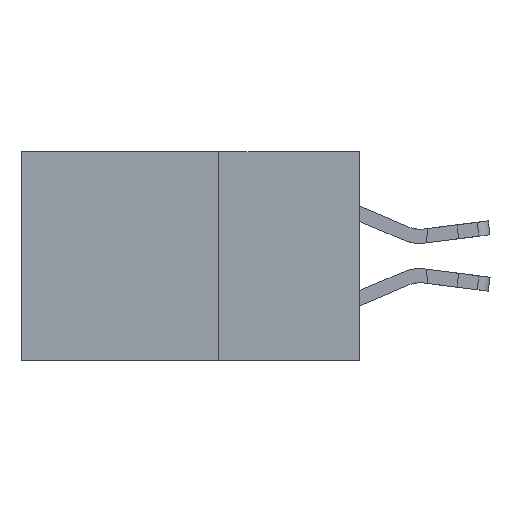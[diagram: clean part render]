
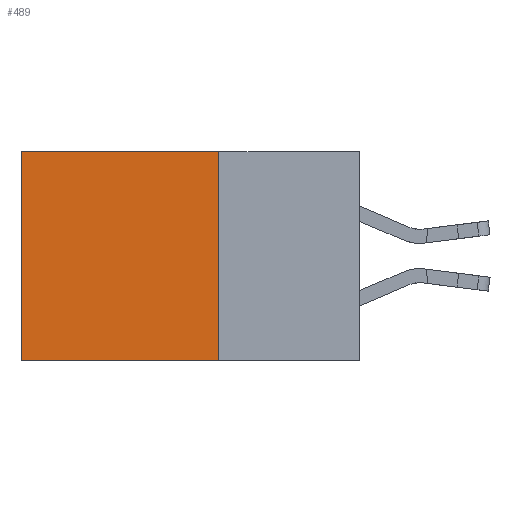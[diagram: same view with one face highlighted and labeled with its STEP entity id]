
A CAD part, left-side view. The second image highlights one B-rep face of the part: STEP entity #489.
In plain terms, the highlighted planar face has unit normal (-1, 0, 0).
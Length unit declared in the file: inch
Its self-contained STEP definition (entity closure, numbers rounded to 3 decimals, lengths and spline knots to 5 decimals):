
#489 = ADVANCED_FACE ( 'NONE', ( #14061 ), #24746, .F. ) ;
#1127 = VERTEX_POINT ( 'NONE', #13816 ) ;
#1723 = CARTESIAN_POINT ( 'NONE',  ( 0.2875, 0.6, -0.37 ) ) ;
#1935 = EDGE_CURVE ( 'NONE', #1127, #5653, #5697, .T. ) ;
#2310 = VERTEX_POINT ( 'NONE', #27118 ) ;
#2506 = CARTESIAN_POINT ( 'NONE',  ( 0.2875, 0.6, 0. ) ) ;
#4691 = DIRECTION ( 'NONE',  ( 1., 0., 0. ) ) ;
#5653 = VERTEX_POINT ( 'NONE', #1723 ) ;
#5697 = LINE ( 'NONE', #22703, #21986 ) ;
#6170 = CARTESIAN_POINT ( 'NONE',  ( 0.2875, 0.6, 0. ) ) ;
#6996 = LINE ( 'NONE', #2506, #26040 ) ;
#9971 = CARTESIAN_POINT ( 'NONE',  ( 0.2875, 0.25, 0. ) ) ;
#11275 = DIRECTION ( 'NONE',  ( 0., 0., -1. ) ) ;
#13816 = CARTESIAN_POINT ( 'NONE',  ( 0.2875, 0.25, -0.37 ) ) ;
#13929 = EDGE_CURVE ( 'NONE', #16594, #5653, #6996, .T. ) ;
#14061 = FACE_OUTER_BOUND ( 'NONE', #19094, .T. ) ;
#16207 = AXIS2_PLACEMENT_3D ( 'NONE', #26859, #4691, #11275 ) ;
#16335 = DIRECTION ( 'NONE',  ( 0., 1., 0. ) ) ;
#16493 = DIRECTION ( 'NONE',  ( 0., 0., -1. ) ) ;
#16594 = VERTEX_POINT ( 'NONE', #6170 ) ;
#16774 = CARTESIAN_POINT ( 'NONE',  ( 0.2875, 0.25, 0. ) ) ;
#18007 = DIRECTION ( 'NONE',  ( 0., 0., -1. ) ) ;
#18491 = VECTOR ( 'NONE', #16493, 39.37008 ) ;
#19094 = EDGE_LOOP ( 'NONE', ( #21877, #20025, #27491, #22542 ) ) ;
#19276 = EDGE_CURVE ( 'NONE', #2310, #1127, #20586, .T. ) ;
#19391 = VECTOR ( 'NONE', #16335, 39.37008 ) ;
#20025 = ORIENTED_EDGE ( 'NONE', *, *, #1935, .F. ) ;
#20393 = DIRECTION ( 'NONE',  ( 0., 1., 0. ) ) ;
#20586 = LINE ( 'NONE', #16774, #18491 ) ;
#21877 = ORIENTED_EDGE ( 'NONE', *, *, #13929, .T. ) ;
#21986 = VECTOR ( 'NONE', #20393, 39.37008 ) ;
#22542 = ORIENTED_EDGE ( 'NONE', *, *, #22694, .T. ) ;
#22694 = EDGE_CURVE ( 'NONE', #2310, #16594, #28361, .T. ) ;
#22703 = CARTESIAN_POINT ( 'NONE',  ( 0.2875, 0.25, -0.37 ) ) ;
#24746 = PLANE ( 'NONE',  #16207 ) ;
#26040 = VECTOR ( 'NONE', #18007, 39.37008 ) ;
#26859 = CARTESIAN_POINT ( 'NONE',  ( 0.2875, 0.25, 0. ) ) ;
#27118 = CARTESIAN_POINT ( 'NONE',  ( 0.2875, 0.25, 0. ) ) ;
#27491 = ORIENTED_EDGE ( 'NONE', *, *, #19276, .F. ) ;
#28361 = LINE ( 'NONE', #9971, #19391 ) ;
